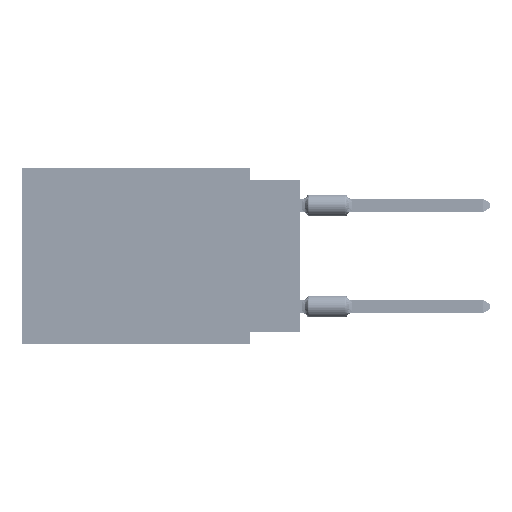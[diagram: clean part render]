
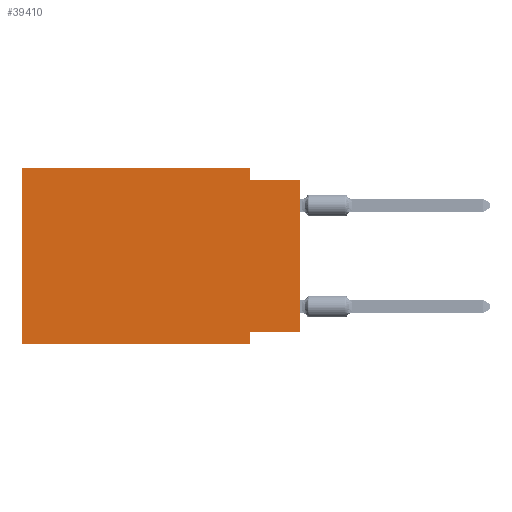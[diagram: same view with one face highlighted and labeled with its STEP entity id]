
A CAD part, left-side view. The second image highlights one B-rep face of the part: STEP entity #39410.
In plain terms, the highlighted planar face has unit normal (-1, 0, 0).
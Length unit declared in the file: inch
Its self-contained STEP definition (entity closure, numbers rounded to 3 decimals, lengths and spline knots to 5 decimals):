
#2108 = DIRECTION ( 'NONE',  ( 0., -1., 0. ) ) ;
#2245 = CARTESIAN_POINT ( 'NONE',  ( 0., 0.1, 0. ) ) ;
#3031 = CARTESIAN_POINT ( 'NONE',  ( 0., 0.1, -0.35 ) ) ;
#3919 = VECTOR ( 'NONE', #11373, 39.37008 ) ;
#6832 = CARTESIAN_POINT ( 'NONE',  ( 0., 0.55, 0. ) ) ;
#8267 = ORIENTED_EDGE ( 'NONE', *, *, #38209, .F. ) ;
#8878 = CARTESIAN_POINT ( 'NONE',  ( 0., 0.1, 0. ) ) ;
#9198 = CARTESIAN_POINT ( 'NONE',  ( 0., 0.1, -0.025 ) ) ;
#9541 = VERTEX_POINT ( 'NONE', #8878 ) ;
#10303 = LINE ( 'NONE', #2245, #103541 ) ;
#11373 = DIRECTION ( 'NONE',  ( 0., 0., 1. ) ) ;
#11646 = EDGE_CURVE ( 'NONE', #99207, #23166, #97425, .T. ) ;
#13355 = DIRECTION ( 'NONE',  ( 0., -1., 0. ) ) ;
#15436 = PLANE ( 'NONE',  #86846 ) ;
#21888 = LINE ( 'NONE', #29462, #32941 ) ;
#23166 = VERTEX_POINT ( 'NONE', #3031 ) ;
#23767 = CARTESIAN_POINT ( 'NONE',  ( 0., 0.55, -0.35 ) ) ;
#27863 = DIRECTION ( 'NONE',  ( 0., 0., -1. ) ) ;
#29462 = CARTESIAN_POINT ( 'NONE',  ( 0., 0.1, -0.35 ) ) ;
#29469 = EDGE_CURVE ( 'NONE', #98292, #66216, #85004, .T. ) ;
#29506 = LINE ( 'NONE', #62281, #35640 ) ;
#32098 = DIRECTION ( 'NONE',  ( 0., -1., 0. ) ) ;
#32941 = VECTOR ( 'NONE', #27863, 39.37008 ) ;
#35370 = CARTESIAN_POINT ( 'NONE',  ( 0., 0., -0.025 ) ) ;
#35640 = VECTOR ( 'NONE', #13355, 39.37008 ) ;
#36877 = EDGE_CURVE ( 'NONE', #48976, #9541, #29506, .T. ) ;
#36902 = LINE ( 'NONE', #38487, #73627 ) ;
#38209 = EDGE_CURVE ( 'NONE', #99207, #48976, #89579, .T. ) ;
#38487 = CARTESIAN_POINT ( 'NONE',  ( 0., 0., -0.325 ) ) ;
#39410 = ADVANCED_FACE ( 'NONE', ( #65392 ), #15436, .F. ) ;
#43301 = EDGE_CURVE ( 'NONE', #93072, #66216, #69252, .T. ) ;
#44990 = EDGE_CURVE ( 'NONE', #98292, #50015, #36902, .T. ) ;
#47366 = CARTESIAN_POINT ( 'NONE',  ( 0., 0., -0.325 ) ) ;
#48669 = CARTESIAN_POINT ( 'NONE',  ( 0., 0.55, -0.35 ) ) ;
#48976 = VERTEX_POINT ( 'NONE', #66218 ) ;
#50015 = VERTEX_POINT ( 'NONE', #62199 ) ;
#50948 = ORIENTED_EDGE ( 'NONE', *, *, #11646, .T. ) ;
#54145 = ORIENTED_EDGE ( 'NONE', *, *, #43301, .F. ) ;
#56282 = CARTESIAN_POINT ( 'NONE',  ( 0., 0., -0.025 ) ) ;
#56801 = DIRECTION ( 'NONE',  ( 1., 0., 0. ) ) ;
#59196 = DIRECTION ( 'NONE',  ( 0., 0., -1. ) ) ;
#59512 = ORIENTED_EDGE ( 'NONE', *, *, #36877, .F. ) ;
#62199 = CARTESIAN_POINT ( 'NONE',  ( 0., 0.1, -0.325 ) ) ;
#62281 = CARTESIAN_POINT ( 'NONE',  ( 0., 0.55, 0. ) ) ;
#62812 = EDGE_CURVE ( 'NONE', #50015, #23166, #21888, .T. ) ;
#64114 = EDGE_CURVE ( 'NONE', #9541, #93072, #10303, .T. ) ;
#64184 = ORIENTED_EDGE ( 'NONE', *, *, #29469, .T. ) ;
#64316 = DIRECTION ( 'NONE',  ( 0., 0., 1. ) ) ;
#65392 = FACE_OUTER_BOUND ( 'NONE', #70489, .T. ) ;
#66216 = VERTEX_POINT ( 'NONE', #35370 ) ;
#66218 = CARTESIAN_POINT ( 'NONE',  ( 0., 0.55, 0. ) ) ;
#68228 = ORIENTED_EDGE ( 'NONE', *, *, #44990, .F. ) ;
#69252 = LINE ( 'NONE', #56282, #85401 ) ;
#70489 = EDGE_LOOP ( 'NONE', ( #64184, #54145, #72652, #59512, #8267, #50948, #78481, #68228 ) ) ;
#71243 = DIRECTION ( 'NONE',  ( 0., 1., 0. ) ) ;
#72652 = ORIENTED_EDGE ( 'NONE', *, *, #64114, .F. ) ;
#73627 = VECTOR ( 'NONE', #71243, 39.37008 ) ;
#78069 = VECTOR ( 'NONE', #64316, 39.37008 ) ;
#78481 = ORIENTED_EDGE ( 'NONE', *, *, #62812, .F. ) ;
#85004 = LINE ( 'NONE', #100086, #3919 ) ;
#85401 = VECTOR ( 'NONE', #32098, 39.37008 ) ;
#86846 = AXIS2_PLACEMENT_3D ( 'NONE', #105209, #56801, #97677 ) ;
#89066 = VECTOR ( 'NONE', #2108, 39.37008 ) ;
#89579 = LINE ( 'NONE', #6832, #78069 ) ;
#93072 = VERTEX_POINT ( 'NONE', #9198 ) ;
#97425 = LINE ( 'NONE', #23767, #89066 ) ;
#97677 = DIRECTION ( 'NONE',  ( 0., 0., -1. ) ) ;
#98292 = VERTEX_POINT ( 'NONE', #47366 ) ;
#99207 = VERTEX_POINT ( 'NONE', #48669 ) ;
#100086 = CARTESIAN_POINT ( 'NONE',  ( 0., 0., 0. ) ) ;
#103541 = VECTOR ( 'NONE', #59196, 39.37008 ) ;
#105209 = CARTESIAN_POINT ( 'NONE',  ( 0., 0.55, 0. ) ) ;
